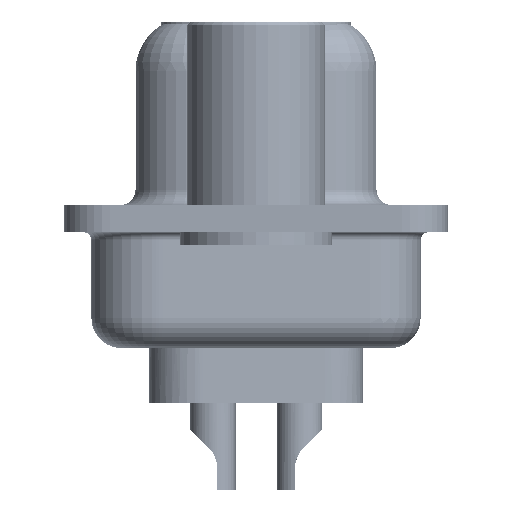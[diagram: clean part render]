
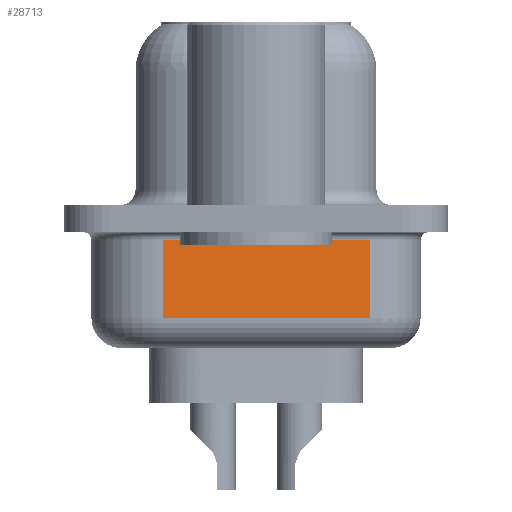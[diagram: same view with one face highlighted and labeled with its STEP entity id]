
A CAD part, left-side view. The second image highlights one B-rep face of the part: STEP entity #28713.
In plain terms, the highlighted planar face has unit normal (-0.985, -0.174, 0).
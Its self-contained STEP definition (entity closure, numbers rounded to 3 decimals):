
#152 = AXIS2_PLACEMENT_3D ( 'NONE', #16195, #23244, #9400 ) ;
#783 = CARTESIAN_POINT ( 'NONE',  ( 4.079, -3.747, -0.7 ) ) ;
#1149 = VECTOR ( 'NONE', #24172, 1000. ) ;
#1705 = EDGE_LOOP ( 'NONE', ( #8426, #11633, #20593, #11235 ) ) ;
#4638 = VECTOR ( 'NONE', #28327, 1000. ) ;
#5631 = VERTEX_POINT ( 'NONE', #6232 ) ;
#6060 = VERTEX_POINT ( 'NONE', #783 ) ;
#6232 = CARTESIAN_POINT ( 'NONE',  ( 2.88, 3.053, -3.25 ) ) ;
#7078 = PLANE ( 'NONE',  #152 ) ;
#7759 = CARTESIAN_POINT ( 'NONE',  ( 2.88, 3.053, -4.25 ) ) ;
#8426 = ORIENTED_EDGE ( 'NONE', *, *, #18352, .F. ) ;
#9300 = DIRECTION ( 'NONE',  ( -0.174, 0.985, 0. ) ) ;
#9400 = DIRECTION ( 'NONE',  ( -0.174, 0.985, 0. ) ) ;
#9774 = CARTESIAN_POINT ( 'NONE',  ( 4.079, -3.747, -4.25 ) ) ;
#11235 = ORIENTED_EDGE ( 'NONE', *, *, #20498, .T. ) ;
#11633 = ORIENTED_EDGE ( 'NONE', *, *, #28360, .T. ) ;
#12976 = EDGE_CURVE ( 'NONE', #14025, #6060, #17560, .T. ) ;
#14025 = VERTEX_POINT ( 'NONE', #27833 ) ;
#14100 = VECTOR ( 'NONE', #23920, 1000. ) ;
#14586 = LINE ( 'NONE', #25446, #20759 ) ;
#14670 = CARTESIAN_POINT ( 'NONE',  ( 2.88, 3.053, -0.7 ) ) ;
#14905 = CARTESIAN_POINT ( 'NONE',  ( 2.88, 3.053, -3.25 ) ) ;
#16195 = CARTESIAN_POINT ( 'NONE',  ( 2.88, 3.053, -4.25 ) ) ;
#17560 = LINE ( 'NONE', #9774, #4638 ) ;
#18352 = EDGE_CURVE ( 'NONE', #5631, #28906, #20291, .T. ) ;
#20291 = LINE ( 'NONE', #7759, #14100 ) ;
#20498 = EDGE_CURVE ( 'NONE', #6060, #28906, #14586, .T. ) ;
#20593 = ORIENTED_EDGE ( 'NONE', *, *, #12976, .T. ) ;
#20759 = VECTOR ( 'NONE', #9300, 1000. ) ;
#23244 = DIRECTION ( 'NONE',  ( 0.985, 0.174, 0. ) ) ;
#23920 = DIRECTION ( 'NONE',  ( 0., 0., 1. ) ) ;
#23988 = FACE_OUTER_BOUND ( 'NONE', #1705, .T. ) ;
#24172 = DIRECTION ( 'NONE',  ( 0.174, -0.985, 0. ) ) ;
#25062 = LINE ( 'NONE', #14905, #1149 ) ;
#25446 = CARTESIAN_POINT ( 'NONE',  ( 2.88, 3.053, -0.7 ) ) ;
#27833 = CARTESIAN_POINT ( 'NONE',  ( 4.079, -3.747, -3.25 ) ) ;
#28327 = DIRECTION ( 'NONE',  ( 0., 0., 1. ) ) ;
#28360 = EDGE_CURVE ( 'NONE', #5631, #14025, #25062, .T. ) ;
#28713 = ADVANCED_FACE ( 'NONE', ( #23988 ), #7078, .F. ) ;
#28906 = VERTEX_POINT ( 'NONE', #14670 ) ;
